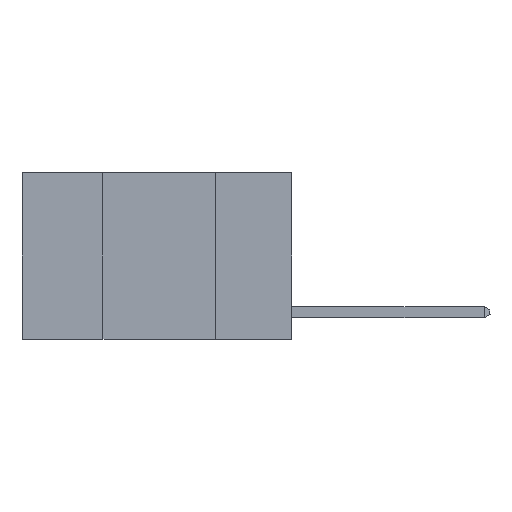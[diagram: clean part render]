
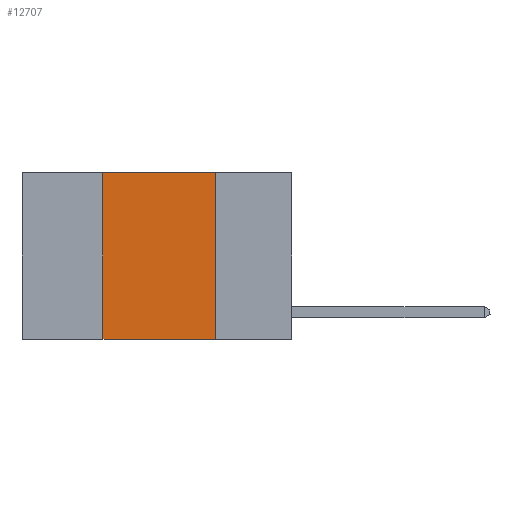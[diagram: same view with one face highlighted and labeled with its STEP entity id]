
A CAD part, left-side view. The second image highlights one B-rep face of the part: STEP entity #12707.
In plain terms, the highlighted planar face has unit normal (-1, 0, 0).
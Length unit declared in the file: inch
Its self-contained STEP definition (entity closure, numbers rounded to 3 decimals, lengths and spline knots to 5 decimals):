
#3175 = DIRECTION ( 'NONE',  ( 0., -1., 0. ) ) ;
#3184 = VECTOR ( 'NONE', #20802, 39.37008 ) ;
#3334 = FACE_OUTER_BOUND ( 'NONE', #8126, .T. ) ;
#4016 = EDGE_CURVE ( 'NONE', #17717, #9382, #20557, .T. ) ;
#4069 = CARTESIAN_POINT ( 'NONE',  ( 0., 0.6, 0. ) ) ;
#4343 = VECTOR ( 'NONE', #14937, 39.37008 ) ;
#4910 = VECTOR ( 'NONE', #3175, 39.37008 ) ;
#4931 = DIRECTION ( 'NONE',  ( 0., -1., 0. ) ) ;
#5271 = ORIENTED_EDGE ( 'NONE', *, *, #8458, .F. ) ;
#5988 = VERTEX_POINT ( 'NONE', #19916 ) ;
#7042 = VERTEX_POINT ( 'NONE', #21931 ) ;
#7092 = DIRECTION ( 'NONE',  ( 1., 0., 0. ) ) ;
#8126 = EDGE_LOOP ( 'NONE', ( #12581, #5271, #21094, #11740 ) ) ;
#8337 = CARTESIAN_POINT ( 'NONE',  ( 0., 0.6, -0.37 ) ) ;
#8458 = EDGE_CURVE ( 'NONE', #9382, #7042, #13560, .T. ) ;
#9201 = PLANE ( 'NONE',  #22445 ) ;
#9382 = VERTEX_POINT ( 'NONE', #23880 ) ;
#9759 = VECTOR ( 'NONE', #4931, 39.37008 ) ;
#10841 = CARTESIAN_POINT ( 'NONE',  ( 0., 0.6, 0. ) ) ;
#10937 = LINE ( 'NONE', #15069, #4343 ) ;
#11740 = ORIENTED_EDGE ( 'NONE', *, *, #17254, .T. ) ;
#12581 = ORIENTED_EDGE ( 'NONE', *, *, #18691, .F. ) ;
#12707 = ADVANCED_FACE ( 'NONE', ( #3334 ), #9201, .F. ) ;
#13560 = LINE ( 'NONE', #4069, #4910 ) ;
#14181 = LINE ( 'NONE', #8337, #9759 ) ;
#14488 = CARTESIAN_POINT ( 'NONE',  ( 0., 0.42, -0.37 ) ) ;
#14937 = DIRECTION ( 'NONE',  ( 0., 0., -1. ) ) ;
#15069 = CARTESIAN_POINT ( 'NONE',  ( 0., 0.17, 0. ) ) ;
#17254 = EDGE_CURVE ( 'NONE', #17717, #5988, #14181, .T. ) ;
#17717 = VERTEX_POINT ( 'NONE', #14488 ) ;
#18691 = EDGE_CURVE ( 'NONE', #7042, #5988, #10937, .T. ) ;
#19916 = CARTESIAN_POINT ( 'NONE',  ( 0., 0.17, -0.37 ) ) ;
#20557 = LINE ( 'NONE', #22818, #3184 ) ;
#20802 = DIRECTION ( 'NONE',  ( 0., 0., 1. ) ) ;
#21094 = ORIENTED_EDGE ( 'NONE', *, *, #4016, .F. ) ;
#21931 = CARTESIAN_POINT ( 'NONE',  ( 0., 0.17, 0. ) ) ;
#22445 = AXIS2_PLACEMENT_3D ( 'NONE', #10841, #7092, #24609 ) ;
#22818 = CARTESIAN_POINT ( 'NONE',  ( 0., 0.42, 0. ) ) ;
#23880 = CARTESIAN_POINT ( 'NONE',  ( 0., 0.42, 0. ) ) ;
#24609 = DIRECTION ( 'NONE',  ( 0., 0., -1. ) ) ;
